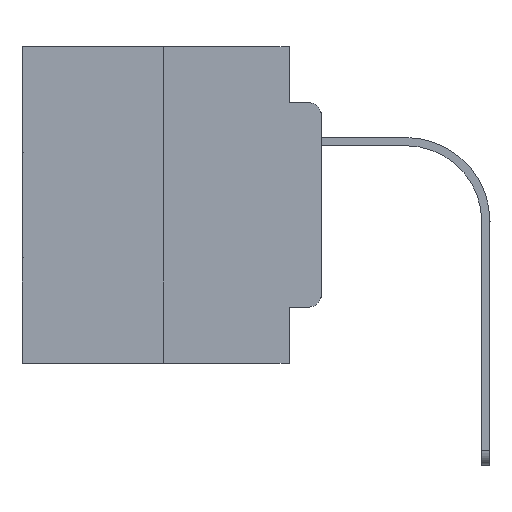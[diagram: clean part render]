
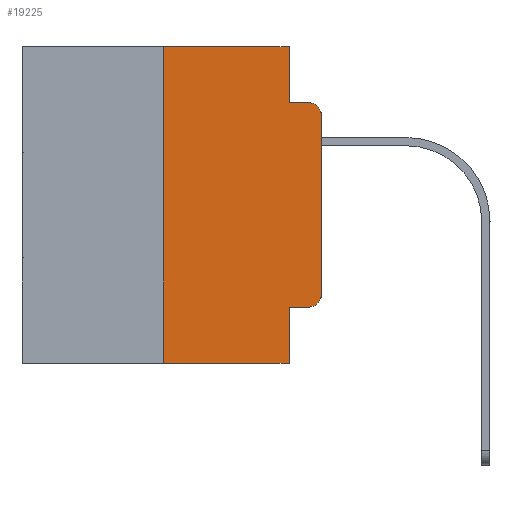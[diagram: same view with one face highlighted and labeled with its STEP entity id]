
A CAD part, left-side view. The second image highlights one B-rep face of the part: STEP entity #19225.
In plain terms, the highlighted planar face has unit normal (-1, 0, 0).
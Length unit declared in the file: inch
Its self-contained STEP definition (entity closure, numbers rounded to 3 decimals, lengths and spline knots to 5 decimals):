
#406 = LINE ( 'NONE', #21002, #17631 ) ;
#424 = DIRECTION ( 'NONE',  ( 0., 0., -1. ) ) ;
#689 = DIRECTION ( 'NONE',  ( -1., 0., 0. ) ) ;
#834 = PLANE ( 'NONE',  #9692 ) ;
#879 = DIRECTION ( 'NONE',  ( 0., 0., 1. ) ) ;
#979 = CARTESIAN_POINT ( 'NONE',  ( 0., 0.473, 0. ) ) ;
#1325 = VECTOR ( 'NONE', #879, 39.37008 ) ;
#1581 = ORIENTED_EDGE ( 'NONE', *, *, #7284, .F. ) ;
#1608 = CARTESIAN_POINT ( 'NONE',  ( 0., 0.051, 0. ) ) ;
#1643 = DIRECTION ( 'NONE',  ( 0., 0., 1. ) ) ;
#2131 = CARTESIAN_POINT ( 'NONE',  ( 0., 0.473, 0. ) ) ;
#2490 = CARTESIAN_POINT ( 'NONE',  ( 0., 0.051, 0. ) ) ;
#3332 = VERTEX_POINT ( 'NONE', #13343 ) ;
#3659 = EDGE_CURVE ( 'NONE', #7542, #8345, #9678, .T. ) ;
#4058 = VECTOR ( 'NONE', #25474, 39.37008 ) ;
#4143 = EDGE_CURVE ( 'NONE', #8345, #9405, #9145, .T. ) ;
#4545 = CARTESIAN_POINT ( 'NONE',  ( 0., 0.051, -0.4115 ) ) ;
#4829 = ORIENTED_EDGE ( 'NONE', *, *, #8187, .T. ) ;
#5012 = ORIENTED_EDGE ( 'NONE', *, *, #4143, .T. ) ;
#5147 = FACE_OUTER_BOUND ( 'NONE', #6269, .T. ) ;
#5638 = DIRECTION ( 'NONE',  ( 0., -1., 0. ) ) ;
#6269 = EDGE_LOOP ( 'NONE', ( #4829, #19919, #24598, #10017, #1581, #17862, #21563, #11906, #7305, #5012 ) ) ;
#6366 = VECTOR ( 'NONE', #1643, 39.37008 ) ;
#7024 = VECTOR ( 'NONE', #18932, 39.37008 ) ;
#7091 = EDGE_CURVE ( 'NONE', #3332, #17611, #406, .T. ) ;
#7284 = EDGE_CURVE ( 'NONE', #17175, #19699, #22079, .T. ) ;
#7305 = ORIENTED_EDGE ( 'NONE', *, *, #3659, .T. ) ;
#7423 = VECTOR ( 'NONE', #11694, 39.37008 ) ;
#7517 = CARTESIAN_POINT ( 'NONE',  ( 0., 0.051, -0.4115 ) ) ;
#7542 = VERTEX_POINT ( 'NONE', #4545 ) ;
#7683 = EDGE_CURVE ( 'NONE', #13232, #20778, #18105, .T. ) ;
#8187 = EDGE_CURVE ( 'NONE', #9405, #13232, #19212, .T. ) ;
#8277 = CARTESIAN_POINT ( 'NONE',  ( 0., 0.02, -0.0885 ) ) ;
#8345 = VERTEX_POINT ( 'NONE', #18538 ) ;
#8985 = CARTESIAN_POINT ( 'NONE',  ( 0., 0., 0. ) ) ;
#8994 = DIRECTION ( 'NONE',  ( 0., 0., -1. ) ) ;
#9071 = AXIS2_PLACEMENT_3D ( 'NONE', #21909, #17343, #8994 ) ;
#9145 = CIRCLE ( 'NONE', #16038, 0.02 ) ;
#9405 = VERTEX_POINT ( 'NONE', #24319 ) ;
#9678 = LINE ( 'NONE', #7517, #7423 ) ;
#9692 = AXIS2_PLACEMENT_3D ( 'NONE', #979, #17545, #19295 ) ;
#10017 = ORIENTED_EDGE ( 'NONE', *, *, #11129, .F. ) ;
#10138 = CARTESIAN_POINT ( 'NONE',  ( 0., 0.051, -0.0885 ) ) ;
#11129 = EDGE_CURVE ( 'NONE', #19699, #18811, #11130, .T. ) ;
#11130 = LINE ( 'NONE', #17314, #4058 ) ;
#11209 = VECTOR ( 'NONE', #5638, 39.37008 ) ;
#11694 = DIRECTION ( 'NONE',  ( 0., -1., 0. ) ) ;
#11906 = ORIENTED_EDGE ( 'NONE', *, *, #16413, .F. ) ;
#13232 = VERTEX_POINT ( 'NONE', #21276 ) ;
#13343 = CARTESIAN_POINT ( 'NONE',  ( 0., 0.25, -0.5 ) ) ;
#14247 = CARTESIAN_POINT ( 'NONE',  ( 0., 0.051, -0.0885 ) ) ;
#16038 = AXIS2_PLACEMENT_3D ( 'NONE', #24903, #689, #424 ) ;
#16413 = EDGE_CURVE ( 'NONE', #7542, #17611, #22949, .T. ) ;
#17175 = VERTEX_POINT ( 'NONE', #22865 ) ;
#17314 = CARTESIAN_POINT ( 'NONE',  ( 0., 0.051, 0. ) ) ;
#17343 = DIRECTION ( 'NONE',  ( -1., 0., 0. ) ) ;
#17545 = DIRECTION ( 'NONE',  ( 1., 0., 0. ) ) ;
#17611 = VERTEX_POINT ( 'NONE', #19066 ) ;
#17631 = VECTOR ( 'NONE', #18989, 39.37008 ) ;
#17833 = CARTESIAN_POINT ( 'NONE',  ( 0., 0.25, 0. ) ) ;
#17862 = ORIENTED_EDGE ( 'NONE', *, *, #20565, .F. ) ;
#18105 = CIRCLE ( 'NONE', #9071, 0.02 ) ;
#18538 = CARTESIAN_POINT ( 'NONE',  ( 0., 0.02, -0.4115 ) ) ;
#18811 = VERTEX_POINT ( 'NONE', #10138 ) ;
#18932 = DIRECTION ( 'NONE',  ( 0., 0., -1. ) ) ;
#18989 = DIRECTION ( 'NONE',  ( 0., -1., 0. ) ) ;
#19066 = CARTESIAN_POINT ( 'NONE',  ( 0., 0.051, -0.5 ) ) ;
#19212 = LINE ( 'NONE', #8985, #1325 ) ;
#19225 = ADVANCED_FACE ( 'NONE', ( #5147 ), #834, .F. ) ;
#19295 = DIRECTION ( 'NONE',  ( 0., 0., -1. ) ) ;
#19699 = VERTEX_POINT ( 'NONE', #1608 ) ;
#19919 = ORIENTED_EDGE ( 'NONE', *, *, #7683, .T. ) ;
#20565 = EDGE_CURVE ( 'NONE', #3332, #17175, #22126, .T. ) ;
#20778 = VERTEX_POINT ( 'NONE', #8277 ) ;
#21002 = CARTESIAN_POINT ( 'NONE',  ( 0., 0.473, -0.5 ) ) ;
#21276 = CARTESIAN_POINT ( 'NONE',  ( 0., 0., -0.1085 ) ) ;
#21563 = ORIENTED_EDGE ( 'NONE', *, *, #7091, .T. ) ;
#21909 = CARTESIAN_POINT ( 'NONE',  ( 0., 0.02, -0.1085 ) ) ;
#22079 = LINE ( 'NONE', #2131, #11209 ) ;
#22126 = LINE ( 'NONE', #17833, #6366 ) ;
#22435 = DIRECTION ( 'NONE',  ( 0., -1., 0. ) ) ;
#22865 = CARTESIAN_POINT ( 'NONE',  ( 0., 0.25, 0. ) ) ;
#22936 = LINE ( 'NONE', #14247, #23883 ) ;
#22949 = LINE ( 'NONE', #2490, #7024 ) ;
#23344 = EDGE_CURVE ( 'NONE', #18811, #20778, #22936, .T. ) ;
#23883 = VECTOR ( 'NONE', #22435, 39.37008 ) ;
#24319 = CARTESIAN_POINT ( 'NONE',  ( 0., 0., -0.3915 ) ) ;
#24598 = ORIENTED_EDGE ( 'NONE', *, *, #23344, .F. ) ;
#24903 = CARTESIAN_POINT ( 'NONE',  ( 0., 0.02, -0.3915 ) ) ;
#25474 = DIRECTION ( 'NONE',  ( 0., 0., -1. ) ) ;
